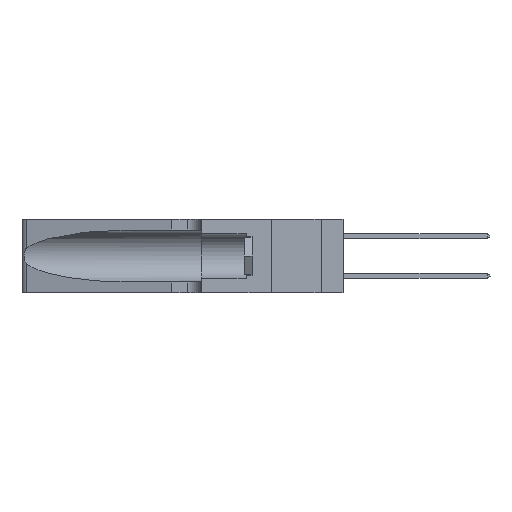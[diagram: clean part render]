
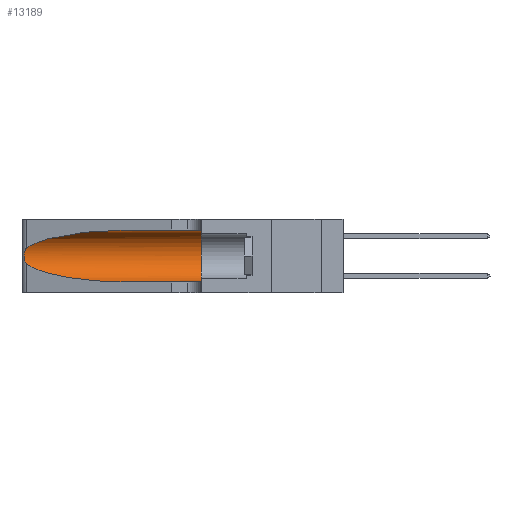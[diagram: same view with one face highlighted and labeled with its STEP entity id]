
A CAD part, left-side view. The second image highlights one B-rep face of the part: STEP entity #13189.
In plain terms, the highlighted cylindrical face has radius 3.308 mm (diameter 6.617 mm), a partial arc.
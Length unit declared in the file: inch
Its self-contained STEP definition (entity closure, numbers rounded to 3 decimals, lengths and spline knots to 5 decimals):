
#395 = DIRECTION ( 'NONE',  ( 0., 0., -1. ) ) ;
#843 = ORIENTED_EDGE ( 'NONE', *, *, #3999, .T. ) ;
#1102 = CARTESIAN_POINT ( 'NONE',  ( 0.1305, 0.72297, 0.31525 ) ) ;
#1217 = CARTESIAN_POINT ( 'NONE',  ( 0.26075, 1.23896, 0.19203 ) ) ;
#1235 = VERTEX_POINT ( 'NONE', #10854 ) ;
#2345 = CARTESIAN_POINT ( 'NONE',  ( 0.25487, 1.22718, 0.14631 ) ) ;
#2841 = CARTESIAN_POINT ( 'NONE',  ( 0.1305, 1.61858, 0.05475 ) ) ;
#3215 = EDGE_LOOP ( 'NONE', ( #23308, #23189, #20390, #843, #29063, #23261 ) ) ;
#3483 = VERTEX_POINT ( 'NONE', #4076 ) ;
#3595 = CARTESIAN_POINT ( 'NONE',  ( 0.2373, 1.15595, 0.28018 ) ) ;
#3999 = EDGE_CURVE ( 'NONE', #1235, #19440, #7447, .T. ) ;
#4076 = CARTESIAN_POINT ( 'NONE',  ( 0.1305, 0.35, 0.31525 ) ) ;
#5812 = EDGE_CURVE ( 'NONE', #24787, #1235, #18120, .T. ) ;
#6156 = CIRCLE ( 'NONE', #14271, 0.13025 ) ;
#6177 = CARTESIAN_POINT ( 'NONE',  ( 0.25555, 1.22993, 0.14849 ) ) ;
#6414 = CARTESIAN_POINT ( 'NONE',  ( 0.26017, 1.23833, 0.17102 ) ) ;
#7447 = LINE ( 'NONE', #2841, #19157 ) ;
#7735 = CARTESIAN_POINT ( 'NONE',  ( 0.2373, 1.15595, 0.08982 ) ) ;
#8665 = DIRECTION ( 'NONE',  ( 0., 1., 0. ) ) ;
#9195 = CARTESIAN_POINT ( 'NONE',  ( 0.25789, 1.23486, 0.15765 ) ) ;
#9771 = EDGE_CURVE ( 'NONE', #3483, #19440, #6156, .T. ) ;
#10854 = CARTESIAN_POINT ( 'NONE',  ( 0.1305, 0.72297, 0.05475 ) ) ;
#11584 = FACE_OUTER_BOUND ( 'NONE', #3215, .T. ) ;
#11681 = CARTESIAN_POINT ( 'NONE',  ( 0.25487, 1.22718, 0.22369 ) ) ;
#13189 = ADVANCED_FACE ( 'NONE', ( #11584 ), #34542, .F. ) ;
#13388 = B_SPLINE_CURVE_WITH_KNOTS ( 'NONE', 3,
 ( #11681, #19489, #24856, #17290, #14348, #22404, #1217, #19726, #6414, #25211, #9195, #17165, #6177, #27551 ),
 .UNSPECIFIED., .F., .F.,
 ( 4, 2, 2, 2, 2, 2, 4 ),
 ( 0., 0.00027, 0.00053, 0.00107, 0.0016, 0.00187, 0.00214 ),
 .UNSPECIFIED. ) ;
#14271 = AXIS2_PLACEMENT_3D ( 'NONE', #19314, #8665, #27353 ) ;
#14348 = CARTESIAN_POINT ( 'NONE',  ( 0.25854, 1.2359, 0.20912 ) ) ;
#14487 = EDGE_CURVE ( 'NONE', #20113, #24551, #27522, .T. ) ;
#14662 = CARTESIAN_POINT ( 'NONE',  ( 0.1305, 1.61858, 0.31525 ) ) ;
#15171 = CARTESIAN_POINT ( 'NONE',  ( 0.25487, 1.22718, 0.14631 ) ) ;
#16590 = CARTESIAN_POINT ( 'NONE',  ( 0.1305, 1.61858, 0.185 ) ) ;
#17139 = DIRECTION ( 'NONE',  ( 0., -1., 0. ) ) ;
#17165 = CARTESIAN_POINT ( 'NONE',  ( 0.25639, 1.23186, 0.15144 ) ) ;
#17290 = CARTESIAN_POINT ( 'NONE',  ( 0.25787, 1.23484, 0.2124 ) ) ;
#18120 =( BOUNDED_CURVE ( )  B_SPLINE_CURVE ( 3, ( #2345, #7735, #24427, #29672 ),
 .UNSPECIFIED., .F., .F. ) 
 B_SPLINE_CURVE_WITH_KNOTS ( ( 4, 4 ),
 ( 3.44316, 4.71239 ),
 .UNSPECIFIED. ) 
 CURVE ( )  GEOMETRIC_REPRESENTATION_ITEM ( )  RATIONAL_B_SPLINE_CURVE ( ( 1., 0.87, 0.87, 1. ) ) 
 REPRESENTATION_ITEM ( '' )  );
#19157 = VECTOR ( 'NONE', #29268, 39.37008 ) ;
#19314 = CARTESIAN_POINT ( 'NONE',  ( 0.1305, 0.35, 0.185 ) ) ;
#19440 = VERTEX_POINT ( 'NONE', #26219 ) ;
#19489 = CARTESIAN_POINT ( 'NONE',  ( 0.25555, 1.22994, 0.2215 ) ) ;
#19726 = CARTESIAN_POINT ( 'NONE',  ( 0.26075, 1.23896, 0.178 ) ) ;
#19845 = CARTESIAN_POINT ( 'NONE',  ( 0.18966, 0.96281, 0.31525 ) ) ;
#20113 = VERTEX_POINT ( 'NONE', #29088 ) ;
#20390 = ORIENTED_EDGE ( 'NONE', *, *, #5812, .T. ) ;
#22404 = CARTESIAN_POINT ( 'NONE',  ( 0.26018, 1.23835, 0.19895 ) ) ;
#23189 = ORIENTED_EDGE ( 'NONE', *, *, #30510, .T. ) ;
#23261 = ORIENTED_EDGE ( 'NONE', *, *, #25285, .F. ) ;
#23308 = ORIENTED_EDGE ( 'NONE', *, *, #14487, .T. ) ;
#23650 = LINE ( 'NONE', #14662, #24476 ) ;
#24427 = CARTESIAN_POINT ( 'NONE',  ( 0.18966, 0.96281, 0.05475 ) ) ;
#24476 = VECTOR ( 'NONE', #17139, 39.37008 ) ;
#24551 = VERTEX_POINT ( 'NONE', #28019 ) ;
#24787 = VERTEX_POINT ( 'NONE', #15171 ) ;
#24856 = CARTESIAN_POINT ( 'NONE',  ( 0.25639, 1.23184, 0.21858 ) ) ;
#25211 = CARTESIAN_POINT ( 'NONE',  ( 0.25856, 1.23593, 0.16098 ) ) ;
#25285 = EDGE_CURVE ( 'NONE', #20113, #3483, #23650, .T. ) ;
#26219 = CARTESIAN_POINT ( 'NONE',  ( 0.1305, 0.35, 0.05475 ) ) ;
#26972 = DIRECTION ( 'NONE',  ( 0., -1., 0. ) ) ;
#27310 = AXIS2_PLACEMENT_3D ( 'NONE', #16590, #26972, #395 ) ;
#27353 = DIRECTION ( 'NONE',  ( 0., 0., 1. ) ) ;
#27522 =( BOUNDED_CURVE ( )  B_SPLINE_CURVE ( 3, ( #1102, #19845, #3595, #30574 ),
 .UNSPECIFIED., .F., .F. ) 
 B_SPLINE_CURVE_WITH_KNOTS ( ( 4, 4 ),
 ( 1.5708, 2.84003 ),
 .UNSPECIFIED. ) 
 CURVE ( )  GEOMETRIC_REPRESENTATION_ITEM ( )  RATIONAL_B_SPLINE_CURVE ( ( 1., 0.87, 0.87, 1. ) ) 
 REPRESENTATION_ITEM ( '' )  );
#27551 = CARTESIAN_POINT ( 'NONE',  ( 0.25487, 1.22718, 0.14631 ) ) ;
#28019 = CARTESIAN_POINT ( 'NONE',  ( 0.25487, 1.22718, 0.22369 ) ) ;
#29063 = ORIENTED_EDGE ( 'NONE', *, *, #9771, .F. ) ;
#29088 = CARTESIAN_POINT ( 'NONE',  ( 0.1305, 0.72297, 0.31525 ) ) ;
#29268 = DIRECTION ( 'NONE',  ( 0., -1., 0. ) ) ;
#29672 = CARTESIAN_POINT ( 'NONE',  ( 0.1305, 0.72297, 0.05475 ) ) ;
#30510 = EDGE_CURVE ( 'NONE', #24551, #24787, #13388, .T. ) ;
#30574 = CARTESIAN_POINT ( 'NONE',  ( 0.25487, 1.22718, 0.22369 ) ) ;
#34542 = CYLINDRICAL_SURFACE ( 'NONE', #27310, 0.13025 ) ;
